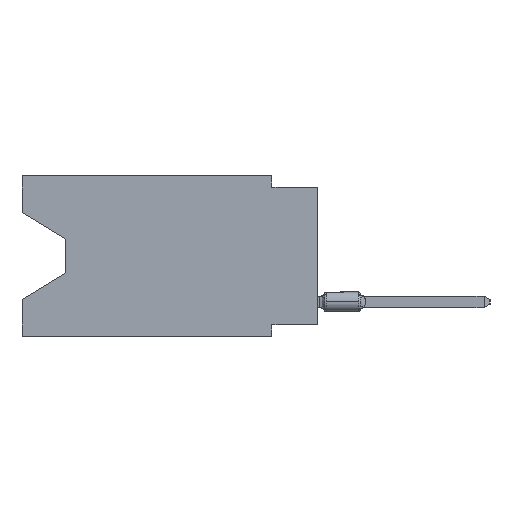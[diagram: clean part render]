
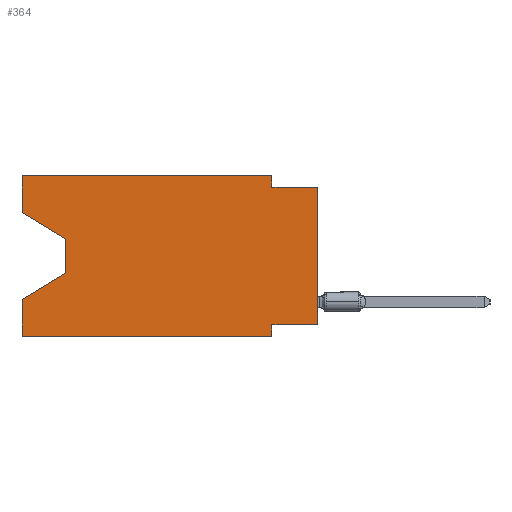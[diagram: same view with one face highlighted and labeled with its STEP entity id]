
A CAD part, left-side view. The second image highlights one B-rep face of the part: STEP entity #364.
In plain terms, the highlighted planar face has unit normal (-1, 0, 0).
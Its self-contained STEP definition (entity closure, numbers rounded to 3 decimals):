
#364 = ADVANCED_FACE ( 'NONE', ( #19613 ), #57497, .F. ) ;
#591 = EDGE_CURVE ( 'NONE', #70087, #30580, #56363, .T. ) ;
#707 = CARTESIAN_POINT ( 'NONE',  ( 0., 2.54, -8.89 ) ) ;
#1193 = CARTESIAN_POINT ( 'NONE',  ( 0., 13.97, -5.385 ) ) ;
#1790 = ORIENTED_EDGE ( 'NONE', *, *, #38117, .F. ) ;
#2340 = ORIENTED_EDGE ( 'NONE', *, *, #2969, .T. ) ;
#2969 = EDGE_CURVE ( 'NONE', #51831, #32146, #6572, .T. ) ;
#4518 = EDGE_CURVE ( 'NONE', #51831, #70087, #18544, .T. ) ;
#4682 = EDGE_CURVE ( 'NONE', #30580, #25702, #41370, .T. ) ;
#5411 = CARTESIAN_POINT ( 'NONE',  ( 0., 13.97, -3.505 ) ) ;
#5451 = ORIENTED_EDGE ( 'NONE', *, *, #45317, .T. ) ;
#5852 = CARTESIAN_POINT ( 'NONE',  ( 0., 16.383, -2.038 ) ) ;
#6572 = LINE ( 'NONE', #5852, #69882 ) ;
#6846 = CARTESIAN_POINT ( 'NONE',  ( 0., 2.54, 0. ) ) ;
#7097 = CARTESIAN_POINT ( 'NONE',  ( 0., 16.383, 0. ) ) ;
#7305 = VECTOR ( 'NONE', #8453, 1000. ) ;
#7972 = VECTOR ( 'NONE', #66621, 1000. ) ;
#8453 = DIRECTION ( 'NONE',  ( 0., 1., 0. ) ) ;
#10081 = LINE ( 'NONE', #5411, #55486 ) ;
#10860 = VERTEX_POINT ( 'NONE', #33925 ) ;
#12703 = CARTESIAN_POINT ( 'NONE',  ( 0., 0., -0.635 ) ) ;
#14144 = EDGE_CURVE ( 'NONE', #39588, #56915, #55382, .T. ) ;
#15238 = CARTESIAN_POINT ( 'NONE',  ( 0., 13.97, -5.385 ) ) ;
#17777 = DIRECTION ( 'NONE',  ( 0., -1., 0. ) ) ;
#18122 = AXIS2_PLACEMENT_3D ( 'NONE', #30339, #52128, #29983 ) ;
#18544 = LINE ( 'NONE', #7097, #18693 ) ;
#18693 = VECTOR ( 'NONE', #45698, 1000. ) ;
#18907 = EDGE_CURVE ( 'NONE', #25702, #35320, #70279, .T. ) ;
#19613 = FACE_OUTER_BOUND ( 'NONE', #61759, .T. ) ;
#20473 = EDGE_CURVE ( 'NONE', #58864, #62189, #21220, .T. ) ;
#21220 = LINE ( 'NONE', #42648, #7305 ) ;
#22094 = DIRECTION ( 'NONE',  ( 0., 0., -1. ) ) ;
#24022 = LINE ( 'NONE', #39063, #34311 ) ;
#25403 = VECTOR ( 'NONE', #43796, 1000. ) ;
#25702 = VERTEX_POINT ( 'NONE', #60161 ) ;
#27109 = CARTESIAN_POINT ( 'NONE',  ( 0., 2.54, -8.89 ) ) ;
#28510 = ORIENTED_EDGE ( 'NONE', *, *, #44346, .F. ) ;
#29983 = DIRECTION ( 'NONE',  ( 0., 0., -1. ) ) ;
#30339 = CARTESIAN_POINT ( 'NONE',  ( 0., 16.383, 0. ) ) ;
#30580 = VERTEX_POINT ( 'NONE', #6846 ) ;
#30707 = CARTESIAN_POINT ( 'NONE',  ( 0., 16.383, -2.038 ) ) ;
#30988 = ORIENTED_EDGE ( 'NONE', *, *, #4682, .F. ) ;
#32146 = VERTEX_POINT ( 'NONE', #32681 ) ;
#32681 = CARTESIAN_POINT ( 'NONE',  ( 0., 13.97, -3.505 ) ) ;
#33925 = CARTESIAN_POINT ( 'NONE',  ( 0., 16.383, -6.852 ) ) ;
#34280 = DIRECTION ( 'NONE',  ( 0., -1., 0. ) ) ;
#34311 = VECTOR ( 'NONE', #66947, 1000. ) ;
#35279 = VERTEX_POINT ( 'NONE', #15238 ) ;
#35320 = VERTEX_POINT ( 'NONE', #12703 ) ;
#35839 = EDGE_CURVE ( 'NONE', #35279, #10860, #65900, .T. ) ;
#38117 = EDGE_CURVE ( 'NONE', #39588, #10860, #59929, .T. ) ;
#39063 = CARTESIAN_POINT ( 'NONE',  ( 0., 0., 0. ) ) ;
#39588 = VERTEX_POINT ( 'NONE', #52021 ) ;
#39825 = DIRECTION ( 'NONE',  ( 0., -0.855, -0.519 ) ) ;
#39828 = VECTOR ( 'NONE', #34280, 1000. ) ;
#41333 = EDGE_CURVE ( 'NONE', #32146, #35279, #10081, .T. ) ;
#41370 = LINE ( 'NONE', #57835, #65474 ) ;
#42648 = CARTESIAN_POINT ( 'NONE',  ( 0., 0., -8.255 ) ) ;
#42727 = CARTESIAN_POINT ( 'NONE',  ( 0., 0., -0.635 ) ) ;
#42761 = CARTESIAN_POINT ( 'NONE',  ( 0., 16.383, 0. ) ) ;
#43584 = ORIENTED_EDGE ( 'NONE', *, *, #41333, .T. ) ;
#43796 = DIRECTION ( 'NONE',  ( 0., -1., 0. ) ) ;
#44346 = EDGE_CURVE ( 'NONE', #62189, #56915, #65335, .T. ) ;
#45317 = EDGE_CURVE ( 'NONE', #58864, #35320, #24022, .T. ) ;
#45334 = CARTESIAN_POINT ( 'NONE',  ( 0., 16.383, -8.89 ) ) ;
#45698 = DIRECTION ( 'NONE',  ( 0., 0., 1. ) ) ;
#50076 = VECTOR ( 'NONE', #17777, 1000. ) ;
#51831 = VERTEX_POINT ( 'NONE', #30707 ) ;
#52021 = CARTESIAN_POINT ( 'NONE',  ( 0., 16.383, -8.89 ) ) ;
#52128 = DIRECTION ( 'NONE',  ( 1., 0., 0. ) ) ;
#52676 = CARTESIAN_POINT ( 'NONE',  ( 0., 16.383, 0. ) ) ;
#53856 = DIRECTION ( 'NONE',  ( 0., 0., 1. ) ) ;
#54116 = ORIENTED_EDGE ( 'NONE', *, *, #14144, .T. ) ;
#55244 = ORIENTED_EDGE ( 'NONE', *, *, #35839, .T. ) ;
#55382 = LINE ( 'NONE', #45334, #39828 ) ;
#55486 = VECTOR ( 'NONE', #59426, 1000. ) ;
#56363 = LINE ( 'NONE', #66750, #50076 ) ;
#56574 = ORIENTED_EDGE ( 'NONE', *, *, #591, .F. ) ;
#56915 = VERTEX_POINT ( 'NONE', #707 ) ;
#57497 = PLANE ( 'NONE',  #18122 ) ;
#57663 = CARTESIAN_POINT ( 'NONE',  ( 0., 0., -8.255 ) ) ;
#57835 = CARTESIAN_POINT ( 'NONE',  ( 0., 2.54, 0. ) ) ;
#58864 = VERTEX_POINT ( 'NONE', #57663 ) ;
#59426 = DIRECTION ( 'NONE',  ( 0., 0., -1. ) ) ;
#59929 = LINE ( 'NONE', #42761, #63265 ) ;
#60161 = CARTESIAN_POINT ( 'NONE',  ( 0., 2.54, -0.635 ) ) ;
#60514 = CARTESIAN_POINT ( 'NONE',  ( 0., 2.54, -8.255 ) ) ;
#61759 = EDGE_LOOP ( 'NONE', ( #2340, #43584, #55244, #1790, #54116, #28510, #70700, #5451, #68275, #30988, #56574, #62114 ) ) ;
#62114 = ORIENTED_EDGE ( 'NONE', *, *, #4518, .F. ) ;
#62189 = VERTEX_POINT ( 'NONE', #60514 ) ;
#63179 = DIRECTION ( 'NONE',  ( 0., 0., -1. ) ) ;
#63265 = VECTOR ( 'NONE', #53856, 1000. ) ;
#63818 = VECTOR ( 'NONE', #22094, 1000. ) ;
#65335 = LINE ( 'NONE', #27109, #63818 ) ;
#65474 = VECTOR ( 'NONE', #63179, 1000. ) ;
#65900 = LINE ( 'NONE', #1193, #7972 ) ;
#66621 = DIRECTION ( 'NONE',  ( 0., 0.855, -0.519 ) ) ;
#66750 = CARTESIAN_POINT ( 'NONE',  ( 0., 16.383, 0. ) ) ;
#66947 = DIRECTION ( 'NONE',  ( 0., 0., 1. ) ) ;
#68275 = ORIENTED_EDGE ( 'NONE', *, *, #18907, .F. ) ;
#69882 = VECTOR ( 'NONE', #39825, 1000. ) ;
#70087 = VERTEX_POINT ( 'NONE', #52676 ) ;
#70279 = LINE ( 'NONE', #42727, #25403 ) ;
#70700 = ORIENTED_EDGE ( 'NONE', *, *, #20473, .F. ) ;
